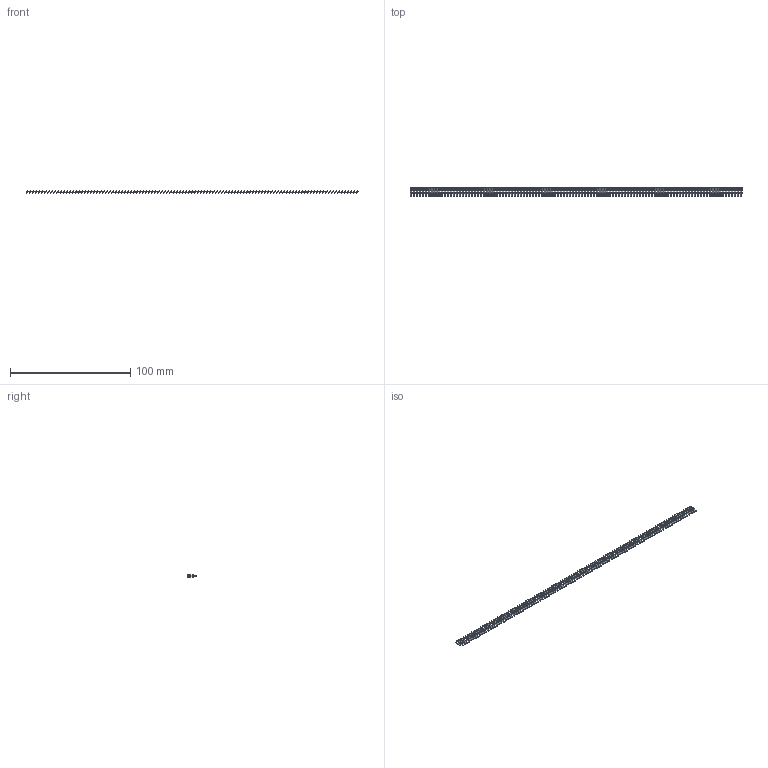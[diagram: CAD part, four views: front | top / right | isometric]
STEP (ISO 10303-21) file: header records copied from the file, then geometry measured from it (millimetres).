
FILE_DESCRIPTION (( 'STEP AP203' ), '1' );
FILE_NAME ('106-109-253-100.STEP', '2020-04-16T23:34:42', ( '' ), ( '' ), 'SwSTEP 2.0', 'SolidWorks 2016', '' );
FILE_SCHEMA (( 'CONFIG_CONTROL_DESIGN' ));
Length unit declared in the file: inch
Products named in the file (2): 106-109-253-100; 100-290-001_100-290-253
Assembly tree (109 placements, depth 2):
  106-109-253-100
    100-290-001_100-290-253  x109
Bounding box: 276.12 x 7.62 x 1.8 mm (x, y, z)
Volume: 601.4 mm3; surface area: 3750.4 mm2
Topology: 109 solids, 109 shells, 2180 faces, 5886 edges, 3924 vertices
Faces by surface type: plane 2071, cylinder 109
Entity records: 4276 total; most frequent: DIRECTION 320, DATE_AND_TIME 228, LOCAL_TIME 228, CALENDAR_DATE 228, COORDINATED_UNIVERSAL_TIME_OFFSET 228, CARTESIAN_POINT 222, AXIS2_PLACEMENT_3D 134, PERSON_AND_ORGANIZATION 125
